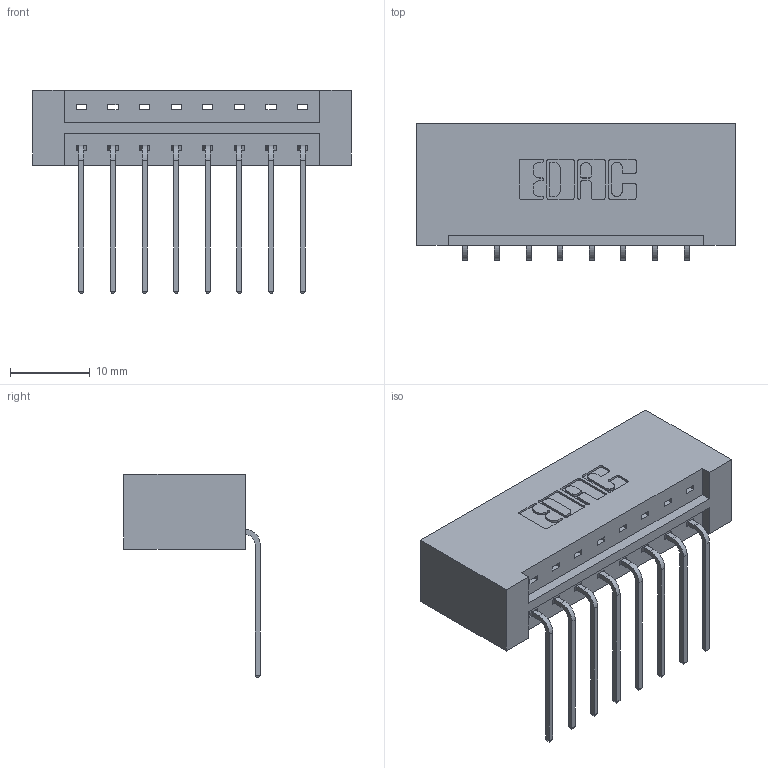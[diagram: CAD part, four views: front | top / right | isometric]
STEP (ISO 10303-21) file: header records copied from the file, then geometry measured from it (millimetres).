
FILE_DESCRIPTION (( 'STEP AP203' ), '1' );
FILE_NAME ('833-008-559-101.STEP', '2020-05-30T16:37:46', ( '' ), ( '' ), 'SwSTEP 2.0', 'SolidWorks 2020', '' );
FILE_SCHEMA (( 'CONFIG_CONTROL_DESIGN' ));
Length unit declared in the file: inch
Products named in the file (3): 833-008-559-101; 345-292-001_558 559 Tail - 1; 833 Part_Lugless
Assembly tree (9 placements, depth 2):
  833-008-559-101
    833 Part_Lugless
    345-292-001_558 559 Tail - 1  x8
Bounding box: 39.95 x 17.09 x 25.53 mm (x, y, z)
Volume: 4367.5 mm3; surface area: 4623 mm2
Topology: 9 solids, 9 shells, 586 faces, 1743 edges, 1150 vertices
Faces by surface type: plane 418, cylinder 168
Entity records: 9095 total; most frequent: CARTESIAN_POINT 1582, ORIENTED_EDGE 1526, DIRECTION 1395, EDGE_CURVE 763, VECTOR 643, LINE 643, VERTEX_POINT 506, AXIS2_PLACEMENT_3D 376
